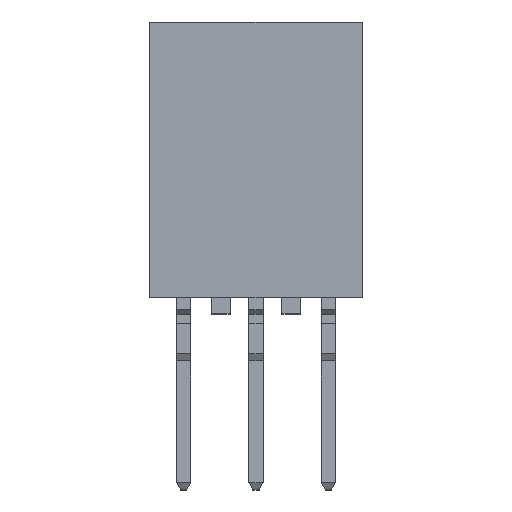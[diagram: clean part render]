
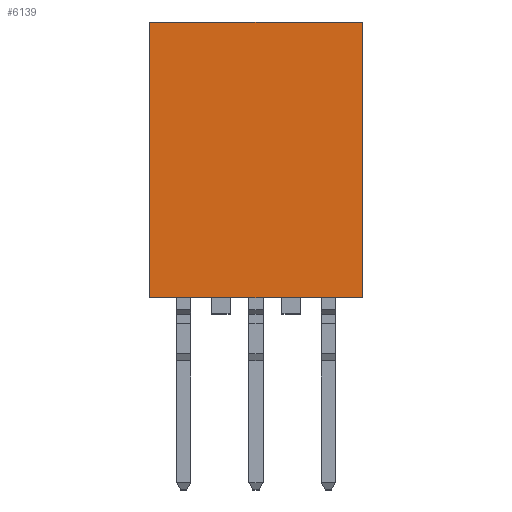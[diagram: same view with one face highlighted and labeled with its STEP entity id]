
A CAD part, top view. The second image highlights one B-rep face of the part: STEP entity #6139.
In plain terms, the highlighted planar face has unit normal (0, 0, 1).
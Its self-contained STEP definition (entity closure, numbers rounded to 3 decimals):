
#148 = DIRECTION ( 'NONE',  ( 1., 0., 0. ) ) ;
#157 = CARTESIAN_POINT ( 'NONE',  ( 8.712, 0., 4.953 ) ) ;
#426 = LINE ( 'NONE', #7845, #7547 ) ;
#604 = AXIS2_PLACEMENT_3D ( 'NONE', #3068, #1683, #7676 ) ;
#751 = EDGE_CURVE ( 'NONE', #6176, #5786, #6547, .T. ) ;
#888 = VECTOR ( 'NONE', #148, 1000. ) ;
#929 = ORIENTED_EDGE ( 'NONE', *, *, #3779, .F. ) ;
#1277 = ORIENTED_EDGE ( 'NONE', *, *, #8437, .F. ) ;
#1683 = DIRECTION ( 'NONE',  ( 0., 0., -1. ) ) ;
#1716 = DIRECTION ( 'NONE',  ( 0., -1., 0. ) ) ;
#2575 = VERTEX_POINT ( 'NONE', #8745 ) ;
#2724 = DIRECTION ( 'NONE',  ( -1., 0., 0. ) ) ;
#2816 = CARTESIAN_POINT ( 'NONE',  ( -4.75, 15.113, 4.953 ) ) ;
#3068 = CARTESIAN_POINT ( 'NONE',  ( -4.75, 15.113, 4.953 ) ) ;
#3196 = DIRECTION ( 'NONE',  ( 0., -1., 0. ) ) ;
#3336 = VECTOR ( 'NONE', #2724, 1000. ) ;
#3779 = EDGE_CURVE ( 'NONE', #2575, #7651, #426, .T. ) ;
#4402 = CARTESIAN_POINT ( 'NONE',  ( -2.921, 15.113, 4.953 ) ) ;
#5124 = CARTESIAN_POINT ( 'NONE',  ( -2.921, 15.113, 4.953 ) ) ;
#5297 = ORIENTED_EDGE ( 'NONE', *, *, #751, .T. ) ;
#5786 = VERTEX_POINT ( 'NONE', #8409 ) ;
#6139 = ADVANCED_FACE ( 'NONE', ( #7767 ), #8528, .F. ) ;
#6176 = VERTEX_POINT ( 'NONE', #5124 ) ;
#6547 = LINE ( 'NONE', #4402, #7271 ) ;
#6806 = LINE ( 'NONE', #2816, #888 ) ;
#6844 = EDGE_CURVE ( 'NONE', #6176, #2575, #6806, .T. ) ;
#6883 = CARTESIAN_POINT ( 'NONE',  ( -4.75, 0., 4.953 ) ) ;
#7002 = EDGE_LOOP ( 'NONE', ( #1277, #929, #8523, #5297 ) ) ;
#7271 = VECTOR ( 'NONE', #3196, 1000. ) ;
#7547 = VECTOR ( 'NONE', #1716, 1000. ) ;
#7651 = VERTEX_POINT ( 'NONE', #157 ) ;
#7676 = DIRECTION ( 'NONE',  ( -1., 0., 0. ) ) ;
#7767 = FACE_OUTER_BOUND ( 'NONE', #7002, .T. ) ;
#7845 = CARTESIAN_POINT ( 'NONE',  ( 8.712, 15.113, 4.953 ) ) ;
#8229 = LINE ( 'NONE', #6883, #3336 ) ;
#8409 = CARTESIAN_POINT ( 'NONE',  ( -2.921, 0., 4.953 ) ) ;
#8437 = EDGE_CURVE ( 'NONE', #7651, #5786, #8229, .T. ) ;
#8523 = ORIENTED_EDGE ( 'NONE', *, *, #6844, .F. ) ;
#8528 = PLANE ( 'NONE',  #604 ) ;
#8745 = CARTESIAN_POINT ( 'NONE',  ( 8.712, 15.113, 4.953 ) ) ;
